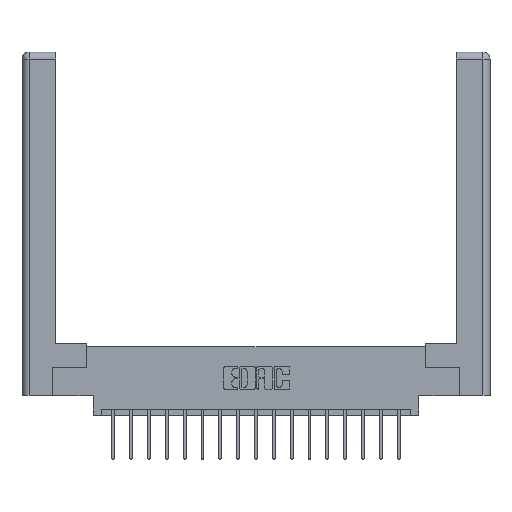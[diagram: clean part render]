
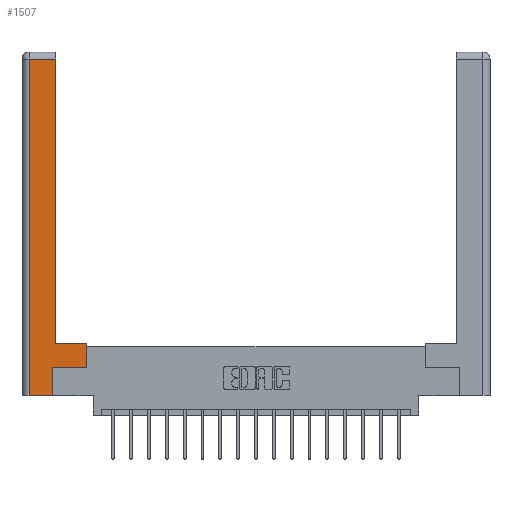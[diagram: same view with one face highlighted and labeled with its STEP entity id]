
A CAD part, top view. The second image highlights one B-rep face of the part: STEP entity #1507.
In plain terms, the highlighted planar face has unit normal (0, 0, 1).
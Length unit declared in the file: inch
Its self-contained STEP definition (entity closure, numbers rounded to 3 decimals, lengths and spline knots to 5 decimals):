
#545 = CARTESIAN_POINT ( 'NONE',  ( 0., 0., 0. ) ) ;
#784 = ORIENTED_EDGE ( 'NONE', *, *, #3002, .T. ) ;
#1105 = CARTESIAN_POINT ( 'NONE',  ( 0.295, 2.94, 0. ) ) ;
#1138 = VECTOR ( 'NONE', #13053, 39.37008 ) ;
#1507 = ADVANCED_FACE ( 'NONE', ( #10420 ), #3640, .F. ) ;
#1633 = CARTESIAN_POINT ( 'NONE',  ( 0.0615, 0., 0. ) ) ;
#1681 = EDGE_CURVE ( 'NONE', #13715, #14014, #9275, .T. ) ;
#1685 = CARTESIAN_POINT ( 'NONE',  ( 0.0615, 2.94, 0. ) ) ;
#2189 = CARTESIAN_POINT ( 'NONE',  ( 0.265, 0., 0. ) ) ;
#2837 = EDGE_CURVE ( 'NONE', #4677, #10621, #6683, .T. ) ;
#3002 = EDGE_CURVE ( 'NONE', #18101, #4677, #6605, .T. ) ;
#3306 = ORIENTED_EDGE ( 'NONE', *, *, #17808, .T. ) ;
#3640 = PLANE ( 'NONE',  #12476 ) ;
#3675 = ORIENTED_EDGE ( 'NONE', *, *, #2837, .T. ) ;
#4473 = DIRECTION ( 'NONE',  ( 0., -1., 0. ) ) ;
#4677 = VERTEX_POINT ( 'NONE', #10770 ) ;
#4919 = CARTESIAN_POINT ( 'NONE',  ( 0.295, 0.45, 0. ) ) ;
#5056 = VECTOR ( 'NONE', #11838, 39.37008 ) ;
#5532 = CARTESIAN_POINT ( 'NONE',  ( 0.265, 0., 0. ) ) ;
#5805 = LINE ( 'NONE', #1633, #15733 ) ;
#5851 = CARTESIAN_POINT ( 'NONE',  ( 0.295, 0.45, 0. ) ) ;
#5913 = DIRECTION ( 'NONE',  ( -1., 0., 0. ) ) ;
#6153 = CARTESIAN_POINT ( 'NONE',  ( 0.265, 0.245, 0. ) ) ;
#6600 = VECTOR ( 'NONE', #11373, 39.37008 ) ;
#6605 = LINE ( 'NONE', #7285, #5056 ) ;
#6683 = LINE ( 'NONE', #5851, #11095 ) ;
#6739 = VECTOR ( 'NONE', #9952, 39.37008 ) ;
#7285 = CARTESIAN_POINT ( 'NONE',  ( 0.565, 0.45, 0. ) ) ;
#7678 = LINE ( 'NONE', #15453, #6739 ) ;
#8496 = DIRECTION ( 'NONE',  ( 1., 0., 0. ) ) ;
#8629 = VERTEX_POINT ( 'NONE', #17761 ) ;
#8686 = DIRECTION ( 'NONE',  ( 1., 0., 0. ) ) ;
#9038 = VERTEX_POINT ( 'NONE', #1105 ) ;
#9275 = LINE ( 'NONE', #5532, #14140 ) ;
#9807 = ORIENTED_EDGE ( 'NONE', *, *, #1681, .T. ) ;
#9952 = DIRECTION ( 'NONE',  ( 0., 1., 0. ) ) ;
#9982 = CARTESIAN_POINT ( 'NONE',  ( 0.565, 0.245, 0. ) ) ;
#9983 = ORIENTED_EDGE ( 'NONE', *, *, #16002, .T. ) ;
#10128 = CARTESIAN_POINT ( 'NONE',  ( 0.295, 3., 0. ) ) ;
#10420 = FACE_OUTER_BOUND ( 'NONE', #17678, .T. ) ;
#10621 = VERTEX_POINT ( 'NONE', #4919 ) ;
#10770 = CARTESIAN_POINT ( 'NONE',  ( 0.565, 0.45, 0. ) ) ;
#10981 = DIRECTION ( 'NONE',  ( -1., 0., 0. ) ) ;
#11095 = VECTOR ( 'NONE', #5913, 39.37008 ) ;
#11373 = DIRECTION ( 'NONE',  ( -1., 0., 0. ) ) ;
#11838 = DIRECTION ( 'NONE',  ( 0., 1., 0. ) ) ;
#11938 = LINE ( 'NONE', #1685, #6600 ) ;
#12061 = LINE ( 'NONE', #10128, #1138 ) ;
#12286 = DIRECTION ( 'NONE',  ( 0., 0., -1. ) ) ;
#12476 = AXIS2_PLACEMENT_3D ( 'NONE', #545, #12286, #10981 ) ;
#12642 = EDGE_CURVE ( 'NONE', #8629, #13715, #5805, .T. ) ;
#13053 = DIRECTION ( 'NONE',  ( 0., 1., 0. ) ) ;
#13273 = LINE ( 'NONE', #14401, #13522 ) ;
#13522 = VECTOR ( 'NONE', #8496, 39.37008 ) ;
#13715 = VERTEX_POINT ( 'NONE', #14700 ) ;
#14014 = VERTEX_POINT ( 'NONE', #2189 ) ;
#14140 = VECTOR ( 'NONE', #8686, 39.37008 ) ;
#14401 = CARTESIAN_POINT ( 'NONE',  ( 0.565, 0.245, 0. ) ) ;
#14510 = ORIENTED_EDGE ( 'NONE', *, *, #14986, .T. ) ;
#14700 = CARTESIAN_POINT ( 'NONE',  ( 0.0615, 0., 0. ) ) ;
#14986 = EDGE_CURVE ( 'NONE', #9038, #8629, #11938, .T. ) ;
#15114 = ORIENTED_EDGE ( 'NONE', *, *, #17082, .T. ) ;
#15219 = ORIENTED_EDGE ( 'NONE', *, *, #12642, .T. ) ;
#15453 = CARTESIAN_POINT ( 'NONE',  ( 0.265, 0.245, 0. ) ) ;
#15733 = VECTOR ( 'NONE', #4473, 39.37008 ) ;
#16002 = EDGE_CURVE ( 'NONE', #16161, #18101, #13273, .T. ) ;
#16161 = VERTEX_POINT ( 'NONE', #6153 ) ;
#17082 = EDGE_CURVE ( 'NONE', #14014, #16161, #7678, .T. ) ;
#17678 = EDGE_LOOP ( 'NONE', ( #3306, #14510, #15219, #9807, #15114, #9983, #784, #3675 ) ) ;
#17761 = CARTESIAN_POINT ( 'NONE',  ( 0.0615, 2.94, 0. ) ) ;
#17808 = EDGE_CURVE ( 'NONE', #10621, #9038, #12061, .T. ) ;
#18101 = VERTEX_POINT ( 'NONE', #9982 ) ;
